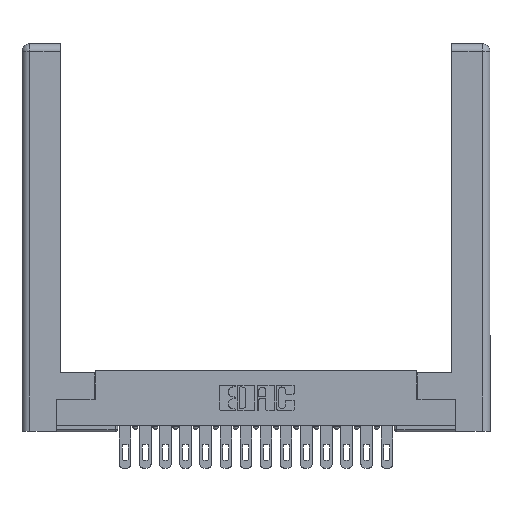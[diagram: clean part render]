
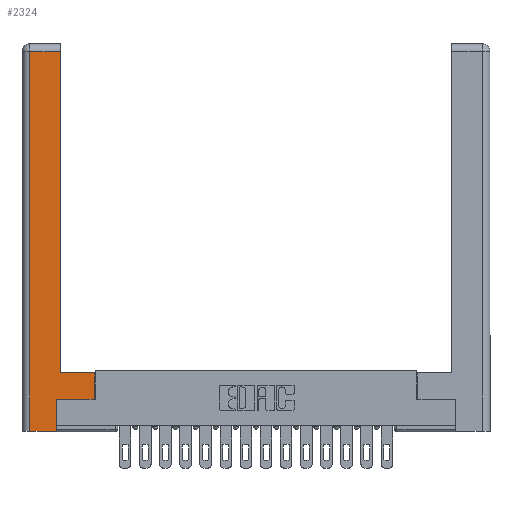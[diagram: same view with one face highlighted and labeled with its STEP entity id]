
A CAD part, top view. The second image highlights one B-rep face of the part: STEP entity #2324.
In plain terms, the highlighted planar face has unit normal (0, 0, 1).
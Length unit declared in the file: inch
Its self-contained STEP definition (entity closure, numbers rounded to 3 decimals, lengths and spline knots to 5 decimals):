
#11 = CARTESIAN_POINT ( 'NONE',  ( 0.565, 0.245, 0. ) ) ;
#21 = DIRECTION ( 'NONE',  ( 1., 0., 0. ) ) ;
#374 = VECTOR ( 'NONE', #1379, 39.37008 ) ;
#799 = VECTOR ( 'NONE', #2846, 39.37008 ) ;
#1028 = LINE ( 'NONE', #10974, #799 ) ;
#1302 = CARTESIAN_POINT ( 'NONE',  ( 0.295, 2.94, 0. ) ) ;
#1379 = DIRECTION ( 'NONE',  ( 0., 1., 0. ) ) ;
#1504 = VERTEX_POINT ( 'NONE', #4692 ) ;
#2178 = LINE ( 'NONE', #6225, #17236 ) ;
#2324 = ADVANCED_FACE ( 'NONE', ( #13610 ), #2641, .F. ) ;
#2641 = PLANE ( 'NONE',  #12240 ) ;
#2846 = DIRECTION ( 'NONE',  ( -1., 0., 0. ) ) ;
#3884 = LINE ( 'NONE', #12469, #4324 ) ;
#3923 = VERTEX_POINT ( 'NONE', #1302 ) ;
#4324 = VECTOR ( 'NONE', #13632, 39.37008 ) ;
#4692 = CARTESIAN_POINT ( 'NONE',  ( 0.295, 0.45, 0. ) ) ;
#5072 = VECTOR ( 'NONE', #6634, 39.37008 ) ;
#5228 = CARTESIAN_POINT ( 'NONE',  ( 0.565, 0.45, 0. ) ) ;
#5298 = DIRECTION ( 'NONE',  ( 1., 0., 0. ) ) ;
#5386 = CARTESIAN_POINT ( 'NONE',  ( 0., 0., 0. ) ) ;
#5415 = EDGE_CURVE ( 'NONE', #14112, #15390, #3884, .T. ) ;
#5457 = CARTESIAN_POINT ( 'NONE',  ( 0.0615, 0., 0. ) ) ;
#5961 = LINE ( 'NONE', #5228, #5072 ) ;
#6154 = LINE ( 'NONE', #10099, #6368 ) ;
#6225 = CARTESIAN_POINT ( 'NONE',  ( 0.295, 0.45, 0. ) ) ;
#6283 = DIRECTION ( 'NONE',  ( -1., 0., 0. ) ) ;
#6368 = VECTOR ( 'NONE', #14422, 39.37008 ) ;
#6634 = DIRECTION ( 'NONE',  ( 0., 1., 0. ) ) ;
#7607 = LINE ( 'NONE', #8323, #374 ) ;
#8278 = EDGE_CURVE ( 'NONE', #3923, #14087, #1028, .T. ) ;
#8280 = ORIENTED_EDGE ( 'NONE', *, *, #5415, .T. ) ;
#8323 = CARTESIAN_POINT ( 'NONE',  ( 0.295, 3., 0. ) ) ;
#8373 = DIRECTION ( 'NONE',  ( 0., 0., -1. ) ) ;
#8387 = EDGE_CURVE ( 'NONE', #13602, #14112, #16938, .T. ) ;
#8578 = ORIENTED_EDGE ( 'NONE', *, *, #11958, .T. ) ;
#9329 = VERTEX_POINT ( 'NONE', #11 ) ;
#10016 = VECTOR ( 'NONE', #5298, 39.37008 ) ;
#10099 = CARTESIAN_POINT ( 'NONE',  ( 0.0615, 0., 0. ) ) ;
#10719 = CARTESIAN_POINT ( 'NONE',  ( 0.565, 0.45, 0. ) ) ;
#10949 = CARTESIAN_POINT ( 'NONE',  ( 0.265, 0., 0. ) ) ;
#10974 = CARTESIAN_POINT ( 'NONE',  ( 0.0615, 2.94, 0. ) ) ;
#11136 = ORIENTED_EDGE ( 'NONE', *, *, #16333, .T. ) ;
#11958 = EDGE_CURVE ( 'NONE', #15390, #9329, #16353, .T. ) ;
#11995 = CARTESIAN_POINT ( 'NONE',  ( 0.0615, 2.94, 0. ) ) ;
#12240 = AXIS2_PLACEMENT_3D ( 'NONE', #5386, #8373, #15249 ) ;
#12469 = CARTESIAN_POINT ( 'NONE',  ( 0.265, 0.245, 0. ) ) ;
#12667 = EDGE_CURVE ( 'NONE', #15025, #1504, #2178, .T. ) ;
#13198 = VECTOR ( 'NONE', #21, 39.37008 ) ;
#13591 = EDGE_CURVE ( 'NONE', #1504, #3923, #7607, .T. ) ;
#13602 = VERTEX_POINT ( 'NONE', #5457 ) ;
#13610 = FACE_OUTER_BOUND ( 'NONE', #16367, .T. ) ;
#13632 = DIRECTION ( 'NONE',  ( 0., 1., 0. ) ) ;
#13871 = ORIENTED_EDGE ( 'NONE', *, *, #13591, .T. ) ;
#14024 = ORIENTED_EDGE ( 'NONE', *, *, #8387, .T. ) ;
#14087 = VERTEX_POINT ( 'NONE', #11995 ) ;
#14112 = VERTEX_POINT ( 'NONE', #10949 ) ;
#14405 = ORIENTED_EDGE ( 'NONE', *, *, #8278, .T. ) ;
#14422 = DIRECTION ( 'NONE',  ( 0., -1., 0. ) ) ;
#15025 = VERTEX_POINT ( 'NONE', #10719 ) ;
#15249 = DIRECTION ( 'NONE',  ( -1., 0., 0. ) ) ;
#15325 = CARTESIAN_POINT ( 'NONE',  ( 0.265, 0., 0. ) ) ;
#15390 = VERTEX_POINT ( 'NONE', #15613 ) ;
#15613 = CARTESIAN_POINT ( 'NONE',  ( 0.265, 0.245, 0. ) ) ;
#16333 = EDGE_CURVE ( 'NONE', #9329, #15025, #5961, .T. ) ;
#16353 = LINE ( 'NONE', #17786, #10016 ) ;
#16367 = EDGE_LOOP ( 'NONE', ( #13871, #14405, #16990, #14024, #8280, #8578, #11136, #17257 ) ) ;
#16938 = LINE ( 'NONE', #15325, #13198 ) ;
#16990 = ORIENTED_EDGE ( 'NONE', *, *, #17744, .T. ) ;
#17236 = VECTOR ( 'NONE', #6283, 39.37008 ) ;
#17257 = ORIENTED_EDGE ( 'NONE', *, *, #12667, .T. ) ;
#17744 = EDGE_CURVE ( 'NONE', #14087, #13602, #6154, .T. ) ;
#17786 = CARTESIAN_POINT ( 'NONE',  ( 0.565, 0.245, 0. ) ) ;
